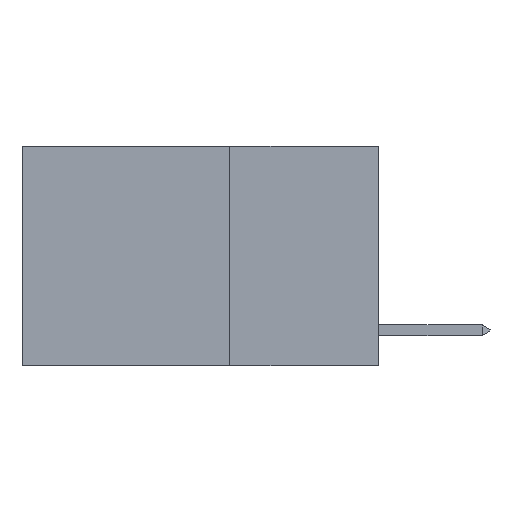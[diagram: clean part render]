
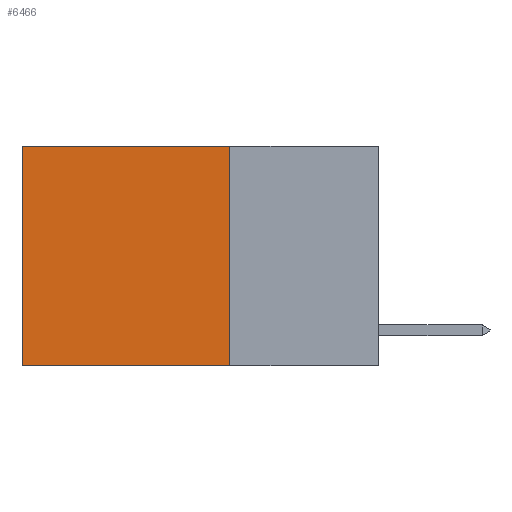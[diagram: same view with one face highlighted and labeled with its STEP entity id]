
A CAD part, left-side view. The second image highlights one B-rep face of the part: STEP entity #6466.
In plain terms, the highlighted planar face has unit normal (-1, 0, 0).
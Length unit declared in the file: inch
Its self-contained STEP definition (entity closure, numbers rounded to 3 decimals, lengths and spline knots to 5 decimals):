
#501 = ORIENTED_EDGE ( 'NONE', *, *, #6469, .T. ) ;
#687 = CARTESIAN_POINT ( 'NONE',  ( 0.2625, 0.25, 0. ) ) ;
#1729 = LINE ( 'NONE', #3404, #7861 ) ;
#1789 = DIRECTION ( 'NONE',  ( 0., 1., 0. ) ) ;
#3210 = EDGE_CURVE ( 'NONE', #5880, #6371, #3759, .T. ) ;
#3256 = VERTEX_POINT ( 'NONE', #4175 ) ;
#3404 = CARTESIAN_POINT ( 'NONE',  ( 0.2625, 0.25, 0. ) ) ;
#3718 = DIRECTION ( 'NONE',  ( 0., 0., -1. ) ) ;
#3759 = LINE ( 'NONE', #6437, #10534 ) ;
#3772 = CARTESIAN_POINT ( 'NONE',  ( 0.2625, 0.6, 0. ) ) ;
#4175 = CARTESIAN_POINT ( 'NONE',  ( 0.2625, 0.6, -0.37 ) ) ;
#4682 = VECTOR ( 'NONE', #3718, 39.37008 ) ;
#5594 = ORIENTED_EDGE ( 'NONE', *, *, #10084, .T. ) ;
#5880 = VERTEX_POINT ( 'NONE', #11269 ) ;
#6371 = VERTEX_POINT ( 'NONE', #6792 ) ;
#6437 = CARTESIAN_POINT ( 'NONE',  ( 0.2625, 0.25, 0. ) ) ;
#6453 = LINE ( 'NONE', #3772, #4682 ) ;
#6466 = ADVANCED_FACE ( 'NONE', ( #9805 ), #9551, .F. ) ;
#6469 = EDGE_CURVE ( 'NONE', #5880, #11411, #1729, .T. ) ;
#6792 = CARTESIAN_POINT ( 'NONE',  ( 0.2625, 0.25, -0.37 ) ) ;
#6952 = VECTOR ( 'NONE', #10127, 39.37008 ) ;
#7335 = EDGE_LOOP ( 'NONE', ( #5594, #11203, #11292, #501 ) ) ;
#7802 = DIRECTION ( 'NONE',  ( 1., 0., 0. ) ) ;
#7861 = VECTOR ( 'NONE', #1789, 39.37008 ) ;
#8012 = CARTESIAN_POINT ( 'NONE',  ( 0.2625, 0.6, 0. ) ) ;
#8230 = AXIS2_PLACEMENT_3D ( 'NONE', #687, #7802, #11368 ) ;
#9551 = PLANE ( 'NONE',  #8230 ) ;
#9805 = FACE_OUTER_BOUND ( 'NONE', #7335, .T. ) ;
#10056 = DIRECTION ( 'NONE',  ( 0., 0., -1. ) ) ;
#10084 = EDGE_CURVE ( 'NONE', #11411, #3256, #6453, .T. ) ;
#10127 = DIRECTION ( 'NONE',  ( 0., 1., 0. ) ) ;
#10534 = VECTOR ( 'NONE', #10056, 39.37008 ) ;
#10938 = LINE ( 'NONE', #10990, #6952 ) ;
#10990 = CARTESIAN_POINT ( 'NONE',  ( 0.2625, 0.25, -0.37 ) ) ;
#11203 = ORIENTED_EDGE ( 'NONE', *, *, #11476, .F. ) ;
#11269 = CARTESIAN_POINT ( 'NONE',  ( 0.2625, 0.25, 0. ) ) ;
#11292 = ORIENTED_EDGE ( 'NONE', *, *, #3210, .F. ) ;
#11368 = DIRECTION ( 'NONE',  ( 0., 0., -1. ) ) ;
#11411 = VERTEX_POINT ( 'NONE', #8012 ) ;
#11476 = EDGE_CURVE ( 'NONE', #6371, #3256, #10938, .T. ) ;
